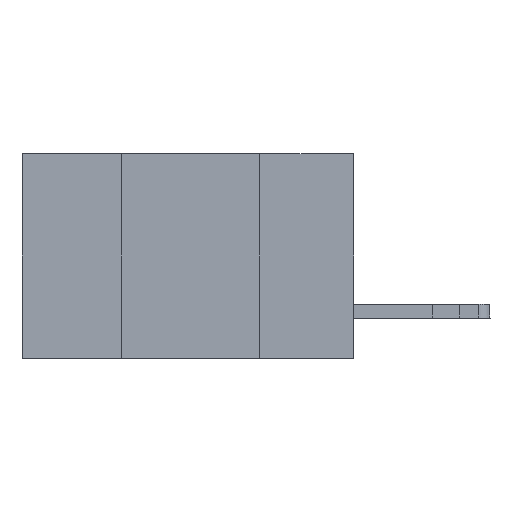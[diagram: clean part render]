
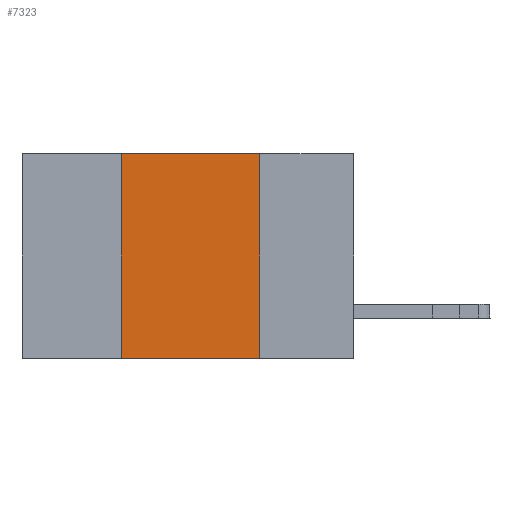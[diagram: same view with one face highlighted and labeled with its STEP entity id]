
A CAD part, left-side view. The second image highlights one B-rep face of the part: STEP entity #7323.
In plain terms, the highlighted planar face has unit normal (-1, 0, 0).
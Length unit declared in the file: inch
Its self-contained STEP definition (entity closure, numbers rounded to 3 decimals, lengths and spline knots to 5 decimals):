
#551 = VERTEX_POINT ( 'NONE', #16708 ) ;
#1571 = LINE ( 'NONE', #11388, #18359 ) ;
#1978 = VECTOR ( 'NONE', #9355, 39.37008 ) ;
#2604 = ORIENTED_EDGE ( 'NONE', *, *, #3043, .F. ) ;
#3043 = EDGE_CURVE ( 'NONE', #3365, #4717, #18871, .T. ) ;
#3365 = VERTEX_POINT ( 'NONE', #18185 ) ;
#4717 = VERTEX_POINT ( 'NONE', #19910 ) ;
#5681 = EDGE_LOOP ( 'NONE', ( #14295, #2604, #11585, #19889 ) ) ;
#5711 = EDGE_CURVE ( 'NONE', #551, #3365, #10456, .T. ) ;
#6892 = PLANE ( 'NONE',  #15864 ) ;
#7323 = ADVANCED_FACE ( 'NONE', ( #17300 ), #6892, .F. ) ;
#8295 = DIRECTION ( 'NONE',  ( 0., 0., -1. ) ) ;
#8480 = DIRECTION ( 'NONE',  ( 1., 0., 0. ) ) ;
#9355 = DIRECTION ( 'NONE',  ( 0., 0., 1. ) ) ;
#10456 = LINE ( 'NONE', #20309, #1978 ) ;
#10810 = CARTESIAN_POINT ( 'NONE',  ( 0., 0.6, 0. ) ) ;
#11388 = CARTESIAN_POINT ( 'NONE',  ( 0., 0.17, 0. ) ) ;
#11467 = VERTEX_POINT ( 'NONE', #12281 ) ;
#11585 = ORIENTED_EDGE ( 'NONE', *, *, #5711, .F. ) ;
#12281 = CARTESIAN_POINT ( 'NONE',  ( 0., 0.17, -0.37 ) ) ;
#12472 = DIRECTION ( 'NONE',  ( 0., -1., 0. ) ) ;
#13154 = EDGE_CURVE ( 'NONE', #4717, #11467, #1571, .T. ) ;
#14295 = ORIENTED_EDGE ( 'NONE', *, *, #13154, .F. ) ;
#14715 = VECTOR ( 'NONE', #12472, 39.37008 ) ;
#15433 = CARTESIAN_POINT ( 'NONE',  ( 0., 0.6, -0.37 ) ) ;
#15864 = AXIS2_PLACEMENT_3D ( 'NONE', #17917, #8480, #19485 ) ;
#16708 = CARTESIAN_POINT ( 'NONE',  ( 0., 0.42, -0.37 ) ) ;
#16970 = VECTOR ( 'NONE', #17014, 39.37008 ) ;
#17014 = DIRECTION ( 'NONE',  ( 0., -1., 0. ) ) ;
#17300 = FACE_OUTER_BOUND ( 'NONE', #5681, .T. ) ;
#17912 = LINE ( 'NONE', #15433, #16970 ) ;
#17917 = CARTESIAN_POINT ( 'NONE',  ( 0., 0.6, 0. ) ) ;
#18185 = CARTESIAN_POINT ( 'NONE',  ( 0., 0.42, 0. ) ) ;
#18359 = VECTOR ( 'NONE', #8295, 39.37008 ) ;
#18774 = EDGE_CURVE ( 'NONE', #551, #11467, #17912, .T. ) ;
#18871 = LINE ( 'NONE', #10810, #14715 ) ;
#19485 = DIRECTION ( 'NONE',  ( 0., 0., -1. ) ) ;
#19889 = ORIENTED_EDGE ( 'NONE', *, *, #18774, .T. ) ;
#19910 = CARTESIAN_POINT ( 'NONE',  ( 0., 0.17, 0. ) ) ;
#20309 = CARTESIAN_POINT ( 'NONE',  ( 0., 0.42, 0. ) ) ;
